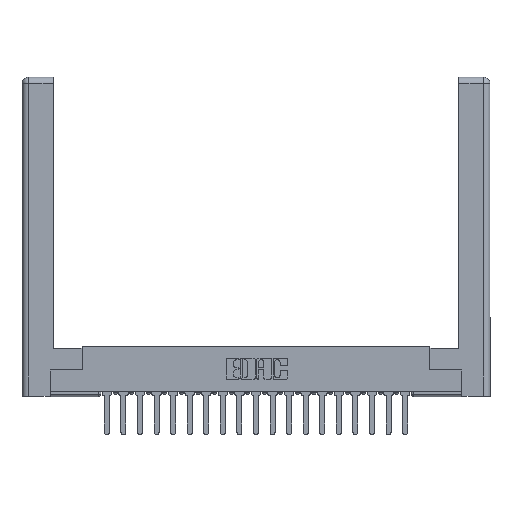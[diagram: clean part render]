
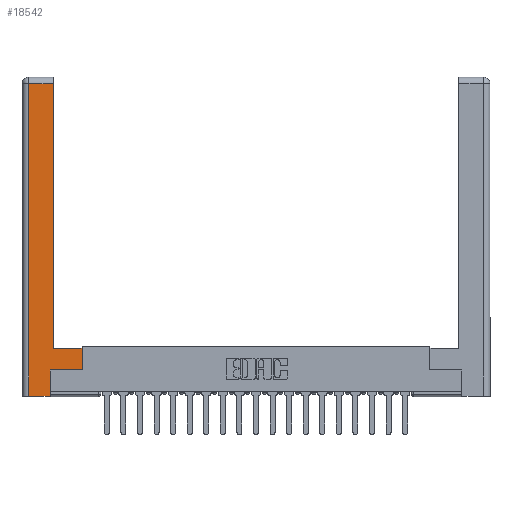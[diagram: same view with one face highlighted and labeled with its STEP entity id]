
A CAD part, top view. The second image highlights one B-rep face of the part: STEP entity #18542.
In plain terms, the highlighted planar face has unit normal (0, 0, 1).
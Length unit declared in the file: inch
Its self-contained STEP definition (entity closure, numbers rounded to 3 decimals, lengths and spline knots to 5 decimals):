
#45 = ORIENTED_EDGE ( 'NONE', *, *, #5635, .T. ) ;
#523 = EDGE_CURVE ( 'NONE', #873, #16694, #7184, .T. ) ;
#873 = VERTEX_POINT ( 'NONE', #4888 ) ;
#1094 = CARTESIAN_POINT ( 'NONE',  ( 0.265, 0.245, 0. ) ) ;
#2854 = CARTESIAN_POINT ( 'NONE',  ( 0.565, 0.245, 0. ) ) ;
#2862 = DIRECTION ( 'NONE',  ( -1., 0., 0. ) ) ;
#2935 = VERTEX_POINT ( 'NONE', #18984 ) ;
#3088 = CARTESIAN_POINT ( 'NONE',  ( 0., 0., 0. ) ) ;
#4017 = EDGE_CURVE ( 'NONE', #15461, #11346, #15835, .T. ) ;
#4738 = EDGE_CURVE ( 'NONE', #11346, #5455, #15223, .T. ) ;
#4888 = CARTESIAN_POINT ( 'NONE',  ( 0.0615, 0., 0. ) ) ;
#5455 = VERTEX_POINT ( 'NONE', #22067 ) ;
#5635 = EDGE_CURVE ( 'NONE', #5455, #2935, #20907, .T. ) ;
#5724 = ORIENTED_EDGE ( 'NONE', *, *, #4738, .T. ) ;
#5769 = VECTOR ( 'NONE', #10316, 39.37008 ) ;
#5980 = DIRECTION ( 'NONE',  ( 0., -1., 0. ) ) ;
#6088 = DIRECTION ( 'NONE',  ( 0., 1., 0. ) ) ;
#6366 = VERTEX_POINT ( 'NONE', #1094 ) ;
#7184 = LINE ( 'NONE', #7406, #7697 ) ;
#7406 = CARTESIAN_POINT ( 'NONE',  ( 0.265, 0., 0. ) ) ;
#7697 = VECTOR ( 'NONE', #17782, 39.37008 ) ;
#7790 = LINE ( 'NONE', #18058, #22199 ) ;
#8219 = CARTESIAN_POINT ( 'NONE',  ( 0.0615, 2.94, 0. ) ) ;
#8534 = ORIENTED_EDGE ( 'NONE', *, *, #4017, .T. ) ;
#8614 = VECTOR ( 'NONE', #21045, 39.37008 ) ;
#9085 = DIRECTION ( 'NONE',  ( -1., 0., 0. ) ) ;
#9642 = DIRECTION ( 'NONE',  ( 0., 0., -1. ) ) ;
#9751 = DIRECTION ( 'NONE',  ( 1., 0., 0. ) ) ;
#9757 = FACE_OUTER_BOUND ( 'NONE', #18438, .T. ) ;
#10316 = DIRECTION ( 'NONE',  ( 0., 1., 0. ) ) ;
#11043 = CARTESIAN_POINT ( 'NONE',  ( 0.565, 0.45, 0. ) ) ;
#11346 = VERTEX_POINT ( 'NONE', #11043 ) ;
#12124 = ORIENTED_EDGE ( 'NONE', *, *, #15819, .T. ) ;
#12174 = EDGE_CURVE ( 'NONE', #16694, #6366, #7790, .T. ) ;
#14124 = CARTESIAN_POINT ( 'NONE',  ( 0.565, 0.45, 0. ) ) ;
#14244 = LINE ( 'NONE', #18094, #18965 ) ;
#14714 = CARTESIAN_POINT ( 'NONE',  ( 0.265, 0., 0. ) ) ;
#14725 = EDGE_CURVE ( 'NONE', #2935, #17710, #14244, .T. ) ;
#14769 = CARTESIAN_POINT ( 'NONE',  ( 0.0615, 0., 0. ) ) ;
#15112 = CARTESIAN_POINT ( 'NONE',  ( 0.295, 0.45, 0. ) ) ;
#15223 = LINE ( 'NONE', #15112, #21201 ) ;
#15325 = ORIENTED_EDGE ( 'NONE', *, *, #12174, .T. ) ;
#15458 = EDGE_CURVE ( 'NONE', #6366, #15461, #18330, .T. ) ;
#15461 = VERTEX_POINT ( 'NONE', #16619 ) ;
#15819 = EDGE_CURVE ( 'NONE', #17710, #873, #21470, .T. ) ;
#15835 = LINE ( 'NONE', #14124, #8614 ) ;
#16440 = VECTOR ( 'NONE', #9751, 39.37008 ) ;
#16619 = CARTESIAN_POINT ( 'NONE',  ( 0.565, 0.245, 0. ) ) ;
#16694 = VERTEX_POINT ( 'NONE', #14714 ) ;
#17710 = VERTEX_POINT ( 'NONE', #8219 ) ;
#17782 = DIRECTION ( 'NONE',  ( 1., 0., 0. ) ) ;
#18058 = CARTESIAN_POINT ( 'NONE',  ( 0.265, 0.245, 0. ) ) ;
#18094 = CARTESIAN_POINT ( 'NONE',  ( 0.0615, 2.94, 0. ) ) ;
#18330 = LINE ( 'NONE', #2854, #16440 ) ;
#18438 = EDGE_LOOP ( 'NONE', ( #45, #21802, #12124, #22064, #15325, #22142, #8534, #5724 ) ) ;
#18542 = ADVANCED_FACE ( 'NONE', ( #9757 ), #18574, .F. ) ;
#18574 = PLANE ( 'NONE',  #20856 ) ;
#18640 = DIRECTION ( 'NONE',  ( -1., 0., 0. ) ) ;
#18965 = VECTOR ( 'NONE', #9085, 39.37008 ) ;
#18984 = CARTESIAN_POINT ( 'NONE',  ( 0.295, 2.94, 0. ) ) ;
#20798 = CARTESIAN_POINT ( 'NONE',  ( 0.295, 3., 0. ) ) ;
#20800 = VECTOR ( 'NONE', #5980, 39.37008 ) ;
#20856 = AXIS2_PLACEMENT_3D ( 'NONE', #3088, #9642, #2862 ) ;
#20907 = LINE ( 'NONE', #20798, #5769 ) ;
#21045 = DIRECTION ( 'NONE',  ( 0., 1., 0. ) ) ;
#21201 = VECTOR ( 'NONE', #18640, 39.37008 ) ;
#21470 = LINE ( 'NONE', #14769, #20800 ) ;
#21802 = ORIENTED_EDGE ( 'NONE', *, *, #14725, .T. ) ;
#22064 = ORIENTED_EDGE ( 'NONE', *, *, #523, .T. ) ;
#22067 = CARTESIAN_POINT ( 'NONE',  ( 0.295, 0.45, 0. ) ) ;
#22142 = ORIENTED_EDGE ( 'NONE', *, *, #15458, .T. ) ;
#22199 = VECTOR ( 'NONE', #6088, 39.37008 ) ;
